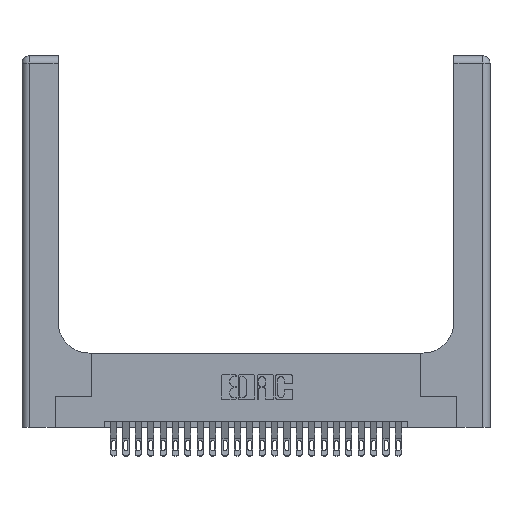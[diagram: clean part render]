
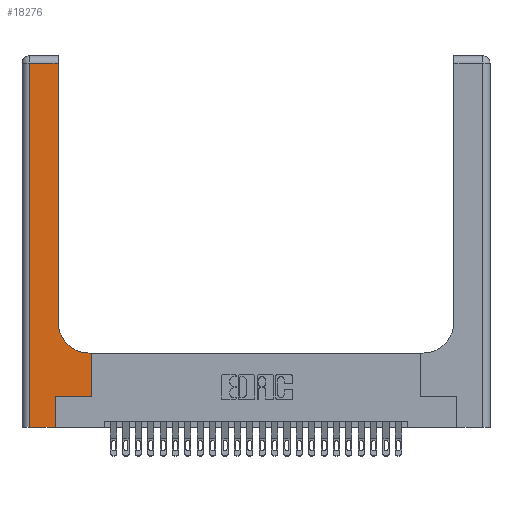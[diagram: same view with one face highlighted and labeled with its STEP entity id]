
A CAD part, top view. The second image highlights one B-rep face of the part: STEP entity #18276.
In plain terms, the highlighted planar face has unit normal (0, 0, 1).
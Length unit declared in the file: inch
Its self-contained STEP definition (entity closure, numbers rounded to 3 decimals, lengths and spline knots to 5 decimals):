
#259 = LINE ( 'NONE', #17746, #2575 ) ;
#691 = VECTOR ( 'NONE', #17312, 39.37008 ) ;
#731 = EDGE_CURVE ( 'NONE', #4303, #4828, #2482, .T. ) ;
#861 = CARTESIAN_POINT ( 'NONE',  ( 0.06, 0., 0.37 ) ) ;
#1141 = CARTESIAN_POINT ( 'NONE',  ( 0.269, 0.25, 0.37 ) ) ;
#1468 = CARTESIAN_POINT ( 'NONE',  ( 0., 2.94, 0.37 ) ) ;
#1491 = DIRECTION ( 'NONE',  ( 0., -1., 0. ) ) ;
#1881 = VERTEX_POINT ( 'NONE', #11617 ) ;
#2441 = DIRECTION ( 'NONE',  ( -1., 0., 0. ) ) ;
#2482 = LINE ( 'NONE', #17908, #17058 ) ;
#2575 = VECTOR ( 'NONE', #21869, 39.37008 ) ;
#3042 = VERTEX_POINT ( 'NONE', #861 ) ;
#3567 = LINE ( 'NONE', #25004, #25162 ) ;
#3738 = VECTOR ( 'NONE', #1491, 39.37008 ) ;
#3852 = ORIENTED_EDGE ( 'NONE', *, *, #16301, .T. ) ;
#4303 = VERTEX_POINT ( 'NONE', #7716 ) ;
#4407 = CARTESIAN_POINT ( 'NONE',  ( 0.2915, 0.6, 0.37 ) ) ;
#4534 = ORIENTED_EDGE ( 'NONE', *, *, #5287, .T. ) ;
#4580 = ORIENTED_EDGE ( 'NONE', *, *, #8590, .T. ) ;
#4828 = VERTEX_POINT ( 'NONE', #25302 ) ;
#5287 = EDGE_CURVE ( 'NONE', #1881, #16028, #22027, .T. ) ;
#5695 = DIRECTION ( 'NONE',  ( 0., 1., 0. ) ) ;
#5733 = EDGE_CURVE ( 'NONE', #11656, #4303, #259, .T. ) ;
#5802 = CARTESIAN_POINT ( 'NONE',  ( 0.269, 0., 0.37 ) ) ;
#6059 = CARTESIAN_POINT ( 'NONE',  ( 0.2915, 0.85, 0.37 ) ) ;
#6856 = DIRECTION ( 'NONE',  ( 0., 0., -1. ) ) ;
#7593 = LINE ( 'NONE', #18326, #3738 ) ;
#7716 = CARTESIAN_POINT ( 'NONE',  ( 0.5585, 0.25, 0.37 ) ) ;
#8167 = VERTEX_POINT ( 'NONE', #6059 ) ;
#8422 = VECTOR ( 'NONE', #24065, 39.37008 ) ;
#8590 = EDGE_CURVE ( 'NONE', #16028, #3042, #7593, .T. ) ;
#8762 = DIRECTION ( 'NONE',  ( 0., 0., -1. ) ) ;
#8973 = CARTESIAN_POINT ( 'NONE',  ( 0.269, 0., 0.37 ) ) ;
#10172 = ORIENTED_EDGE ( 'NONE', *, *, #731, .T. ) ;
#11495 = VERTEX_POINT ( 'NONE', #5802 ) ;
#11617 = CARTESIAN_POINT ( 'NONE',  ( 0.2915, 2.94, 0.37 ) ) ;
#11656 = VERTEX_POINT ( 'NONE', #1141 ) ;
#11715 = LINE ( 'NONE', #8973, #691 ) ;
#12296 = ORIENTED_EDGE ( 'NONE', *, *, #14360, .T. ) ;
#13055 = VERTEX_POINT ( 'NONE', #25586 ) ;
#13574 = LINE ( 'NONE', #4407, #25164 ) ;
#14023 = EDGE_CURVE ( 'NONE', #13055, #8167, #24343, .T. ) ;
#14360 = EDGE_CURVE ( 'NONE', #11495, #11656, #11715, .T. ) ;
#14847 = CARTESIAN_POINT ( 'NONE',  ( 0., 3., 0.37 ) ) ;
#15074 = FACE_OUTER_BOUND ( 'NONE', #24672, .T. ) ;
#16028 = VERTEX_POINT ( 'NONE', #25361 ) ;
#16175 = ORIENTED_EDGE ( 'NONE', *, *, #17988, .T. ) ;
#16301 = EDGE_CURVE ( 'NONE', #4828, #13055, #13574, .T. ) ;
#17058 = VECTOR ( 'NONE', #5695, 39.37008 ) ;
#17312 = DIRECTION ( 'NONE',  ( 0., 1., 0. ) ) ;
#17358 = LINE ( 'NONE', #17862, #23455 ) ;
#17746 = CARTESIAN_POINT ( 'NONE',  ( 0.269, 0.25, 0.37 ) ) ;
#17862 = CARTESIAN_POINT ( 'NONE',  ( 0.2915, 3., 0.37 ) ) ;
#17908 = CARTESIAN_POINT ( 'NONE',  ( 0.5585, 0.25, 0.37 ) ) ;
#17988 = EDGE_CURVE ( 'NONE', #8167, #1881, #17358, .T. ) ;
#18033 = AXIS2_PLACEMENT_3D ( 'NONE', #14847, #8762, #2441 ) ;
#18276 = ADVANCED_FACE ( 'NONE', ( #15074 ), #18991, .F. ) ;
#18326 = CARTESIAN_POINT ( 'NONE',  ( 0.06, 3., 0.37 ) ) ;
#18991 = PLANE ( 'NONE',  #18033 ) ;
#19586 = DIRECTION ( 'NONE',  ( 1., 0., 0. ) ) ;
#19756 = ORIENTED_EDGE ( 'NONE', *, *, #14023, .T. ) ;
#20063 = ORIENTED_EDGE ( 'NONE', *, *, #5733, .T. ) ;
#20081 = DIRECTION ( 'NONE',  ( 0., 1., 0. ) ) ;
#21152 = EDGE_CURVE ( 'NONE', #3042, #11495, #3567, .T. ) ;
#21481 = CARTESIAN_POINT ( 'NONE',  ( 0.5415, 0.85, 0.37 ) ) ;
#21869 = DIRECTION ( 'NONE',  ( 1., 0., 0. ) ) ;
#22027 = LINE ( 'NONE', #1468, #8422 ) ;
#22777 = AXIS2_PLACEMENT_3D ( 'NONE', #21481, #6856, #19586 ) ;
#22850 = DIRECTION ( 'NONE',  ( 1., 0., 0. ) ) ;
#23455 = VECTOR ( 'NONE', #20081, 39.37008 ) ;
#24065 = DIRECTION ( 'NONE',  ( -1., 0., 0. ) ) ;
#24343 = CIRCLE ( 'NONE', #22777, 0.25 ) ;
#24672 = EDGE_LOOP ( 'NONE', ( #16175, #4534, #4580, #26512, #12296, #20063, #10172, #3852, #19756 ) ) ;
#24980 = DIRECTION ( 'NONE',  ( -1., 0., 0. ) ) ;
#25004 = CARTESIAN_POINT ( 'NONE',  ( 0., 0., 0.37 ) ) ;
#25162 = VECTOR ( 'NONE', #22850, 39.37008 ) ;
#25164 = VECTOR ( 'NONE', #24980, 39.37008 ) ;
#25302 = CARTESIAN_POINT ( 'NONE',  ( 0.5585, 0.6, 0.37 ) ) ;
#25361 = CARTESIAN_POINT ( 'NONE',  ( 0.06, 2.94, 0.37 ) ) ;
#25586 = CARTESIAN_POINT ( 'NONE',  ( 0.5415, 0.6, 0.37 ) ) ;
#26512 = ORIENTED_EDGE ( 'NONE', *, *, #21152, .T. ) ;
